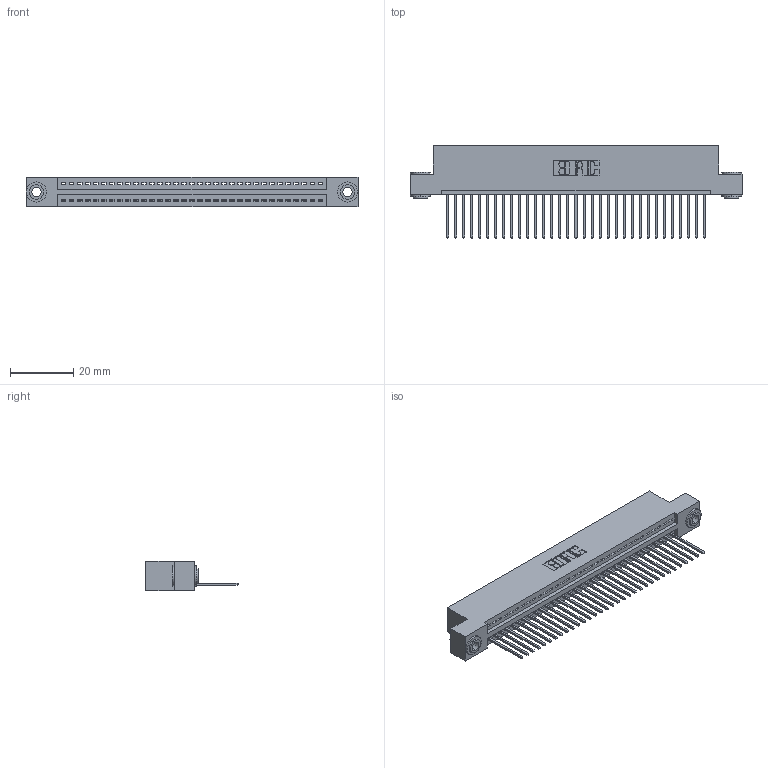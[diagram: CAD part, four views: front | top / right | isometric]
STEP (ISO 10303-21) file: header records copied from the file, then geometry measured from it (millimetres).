
FILE_DESCRIPTION (( 'STEP AP203' ), '1' );
FILE_NAME ('345-033-540-103.STEP', '2018-08-24T11:12:09', ( '' ), ( '' ), 'SwSTEP 2.0', 'SolidWorks 2016', '' );
FILE_SCHEMA (( 'CONFIG_CONTROL_DESIGN' ));
Length unit declared in the file: inch
Products named in the file (4): 345 Part_Flush Mounting Lugs - 0.156 Dia-TH; 345-292-001_345-293-140; 345-250-002_345-250-002-102; 345-033-540-103
Assembly tree (36 placements, depth 2):
  345-033-540-103
    345 Part_Flush Mounting Lugs - 0.156 Dia-TH
    345-292-001_345-293-140  x33
    345-250-002_345-250-002-102  x2
Bounding box: 105.03 x 29.13 x 9.4 mm (x, y, z)
Volume: 9966.1 mm3; surface area: 13657.8 mm2
Topology: 36 solids, 36 shells, 2078 faces, 6225 edges, 4102 vertices
Faces by surface type: plane 1410, cylinder 660, cone 8
Entity records: 26716 total; most frequent: CARTESIAN_POINT 4606, ORIENTED_EDGE 4566, DIRECTION 4067, EDGE_CURVE 2283, VECTOR 1995, LINE 1995, VERTEX_POINT 1518, AXIS2_PLACEMENT_3D 1036
